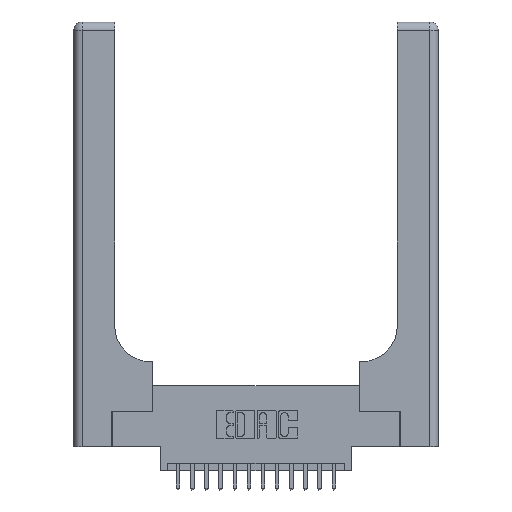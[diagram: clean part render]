
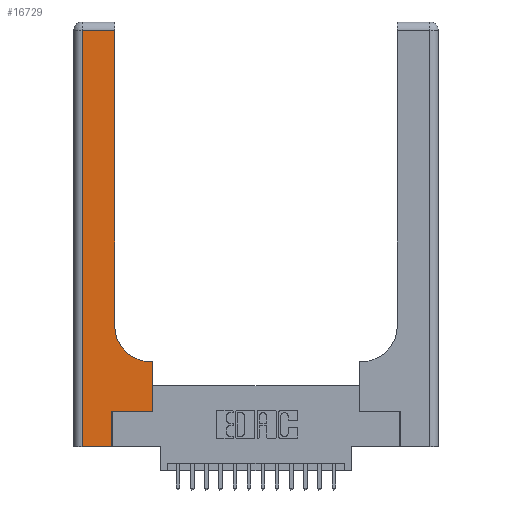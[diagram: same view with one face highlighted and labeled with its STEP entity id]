
A CAD part, top view. The second image highlights one B-rep face of the part: STEP entity #16729.
In plain terms, the highlighted planar face has unit normal (0, 0, 1).
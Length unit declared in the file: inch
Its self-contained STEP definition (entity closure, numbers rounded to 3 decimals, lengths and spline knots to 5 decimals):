
#471 = CARTESIAN_POINT ( 'NONE',  ( 0.5585, 0.25, 0.37 ) ) ;
#577 = EDGE_CURVE ( 'NONE', #9544, #9756, #3196, .T. ) ;
#679 = CARTESIAN_POINT ( 'NONE',  ( 0., 0., 0.37 ) ) ;
#886 = CARTESIAN_POINT ( 'NONE',  ( 0.2915, 2.94, 0.37 ) ) ;
#1058 = VERTEX_POINT ( 'NONE', #3523 ) ;
#1460 = DIRECTION ( 'NONE',  ( 0., 0., -1. ) ) ;
#2551 = LINE ( 'NONE', #4385, #11384 ) ;
#2595 = CARTESIAN_POINT ( 'NONE',  ( 0.2915, 0.6, 0.37 ) ) ;
#2819 = CIRCLE ( 'NONE', #14859, 0.25 ) ;
#2891 = CARTESIAN_POINT ( 'NONE',  ( 0.5415, 0.6, 0.37 ) ) ;
#2928 = VERTEX_POINT ( 'NONE', #16619 ) ;
#3196 = LINE ( 'NONE', #16097, #14998 ) ;
#3352 = DIRECTION ( 'NONE',  ( 0., -1., 0. ) ) ;
#3523 = CARTESIAN_POINT ( 'NONE',  ( 0.269, 0., 0.37 ) ) ;
#3845 = EDGE_CURVE ( 'NONE', #13655, #7123, #2819, .T. ) ;
#4152 = DIRECTION ( 'NONE',  ( 1., 0., 0. ) ) ;
#4385 = CARTESIAN_POINT ( 'NONE',  ( 0.269, 0.25, 0.37 ) ) ;
#4636 = EDGE_CURVE ( 'NONE', #9756, #11307, #8703, .T. ) ;
#4730 = DIRECTION ( 'NONE',  ( 0., 1., 0. ) ) ;
#5161 = VECTOR ( 'NONE', #5252, 39.37008 ) ;
#5252 = DIRECTION ( 'NONE',  ( 0., 1., 0. ) ) ;
#5546 = CARTESIAN_POINT ( 'NONE',  ( 0.2915, 0.85, 0.37 ) ) ;
#6089 = LINE ( 'NONE', #6410, #10619 ) ;
#6280 = ORIENTED_EDGE ( 'NONE', *, *, #14994, .T. ) ;
#6410 = CARTESIAN_POINT ( 'NONE',  ( 0.269, 0., 0.37 ) ) ;
#7123 = VERTEX_POINT ( 'NONE', #5546 ) ;
#7145 = VECTOR ( 'NONE', #3352, 39.37008 ) ;
#7261 = PLANE ( 'NONE',  #11530 ) ;
#7301 = CARTESIAN_POINT ( 'NONE',  ( 0.5585, 0.25, 0.37 ) ) ;
#7502 = EDGE_CURVE ( 'NONE', #11307, #1058, #14400, .T. ) ;
#7524 = ORIENTED_EDGE ( 'NONE', *, *, #577, .T. ) ;
#7930 = CARTESIAN_POINT ( 'NONE',  ( 0.06, 3., 0.37 ) ) ;
#8422 = ORIENTED_EDGE ( 'NONE', *, *, #7502, .T. ) ;
#8703 = LINE ( 'NONE', #7930, #7145 ) ;
#8992 = LINE ( 'NONE', #9749, #5161 ) ;
#9266 = CARTESIAN_POINT ( 'NONE',  ( 0.06, 0., 0.37 ) ) ;
#9544 = VERTEX_POINT ( 'NONE', #886 ) ;
#9749 = CARTESIAN_POINT ( 'NONE',  ( 0.2915, 3., 0.37 ) ) ;
#9756 = VERTEX_POINT ( 'NONE', #12741 ) ;
#9860 = CARTESIAN_POINT ( 'NONE',  ( 0.5415, 0.85, 0.37 ) ) ;
#10100 = DIRECTION ( 'NONE',  ( 0., 0., -1. ) ) ;
#10217 = EDGE_CURVE ( 'NONE', #7123, #9544, #8992, .T. ) ;
#10619 = VECTOR ( 'NONE', #16540, 39.37008 ) ;
#10660 = ORIENTED_EDGE ( 'NONE', *, *, #4636, .T. ) ;
#11307 = VERTEX_POINT ( 'NONE', #9266 ) ;
#11384 = VECTOR ( 'NONE', #17386, 39.37008 ) ;
#11530 = AXIS2_PLACEMENT_3D ( 'NONE', #13254, #1460, #17385 ) ;
#11731 = DIRECTION ( 'NONE',  ( 1., 0., 0. ) ) ;
#12016 = ORIENTED_EDGE ( 'NONE', *, *, #13579, .T. ) ;
#12741 = CARTESIAN_POINT ( 'NONE',  ( 0.06, 2.94, 0.37 ) ) ;
#13073 = EDGE_CURVE ( 'NONE', #2928, #17326, #2551, .T. ) ;
#13254 = CARTESIAN_POINT ( 'NONE',  ( 0., 3., 0.37 ) ) ;
#13579 = EDGE_CURVE ( 'NONE', #14199, #13655, #15466, .T. ) ;
#13655 = VERTEX_POINT ( 'NONE', #2891 ) ;
#13782 = ORIENTED_EDGE ( 'NONE', *, *, #13073, .T. ) ;
#13867 = VECTOR ( 'NONE', #18589, 39.37008 ) ;
#14199 = VERTEX_POINT ( 'NONE', #17476 ) ;
#14200 = ORIENTED_EDGE ( 'NONE', *, *, #3845, .T. ) ;
#14242 = EDGE_LOOP ( 'NONE', ( #18101, #7524, #10660, #8422, #6280, #13782, #15983, #12016, #14200 ) ) ;
#14400 = LINE ( 'NONE', #679, #14615 ) ;
#14427 = EDGE_CURVE ( 'NONE', #17326, #14199, #17470, .T. ) ;
#14432 = FACE_OUTER_BOUND ( 'NONE', #14242, .T. ) ;
#14615 = VECTOR ( 'NONE', #4152, 39.37008 ) ;
#14859 = AXIS2_PLACEMENT_3D ( 'NONE', #9860, #10100, #11731 ) ;
#14994 = EDGE_CURVE ( 'NONE', #1058, #2928, #6089, .T. ) ;
#14998 = VECTOR ( 'NONE', #16783, 39.37008 ) ;
#15466 = LINE ( 'NONE', #2595, #13867 ) ;
#15983 = ORIENTED_EDGE ( 'NONE', *, *, #14427, .T. ) ;
#16097 = CARTESIAN_POINT ( 'NONE',  ( 0., 2.94, 0.37 ) ) ;
#16540 = DIRECTION ( 'NONE',  ( 0., 1., 0. ) ) ;
#16619 = CARTESIAN_POINT ( 'NONE',  ( 0.269, 0.25, 0.37 ) ) ;
#16729 = ADVANCED_FACE ( 'NONE', ( #14432 ), #7261, .F. ) ;
#16783 = DIRECTION ( 'NONE',  ( -1., 0., 0. ) ) ;
#17326 = VERTEX_POINT ( 'NONE', #7301 ) ;
#17385 = DIRECTION ( 'NONE',  ( -1., 0., 0. ) ) ;
#17386 = DIRECTION ( 'NONE',  ( 1., 0., 0. ) ) ;
#17470 = LINE ( 'NONE', #471, #17685 ) ;
#17476 = CARTESIAN_POINT ( 'NONE',  ( 0.5585, 0.6, 0.37 ) ) ;
#17685 = VECTOR ( 'NONE', #4730, 39.37008 ) ;
#18101 = ORIENTED_EDGE ( 'NONE', *, *, #10217, .T. ) ;
#18589 = DIRECTION ( 'NONE',  ( -1., 0., 0. ) ) ;
